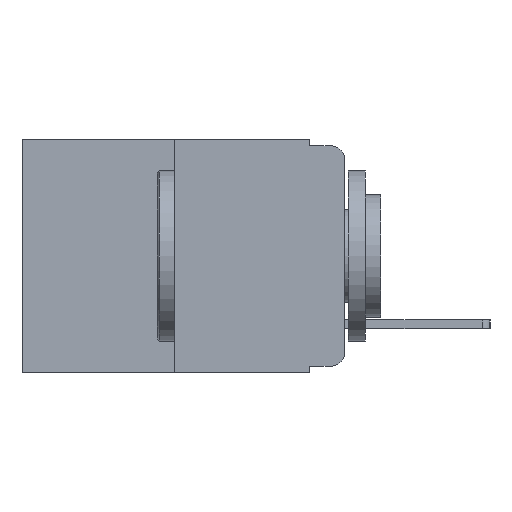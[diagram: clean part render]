
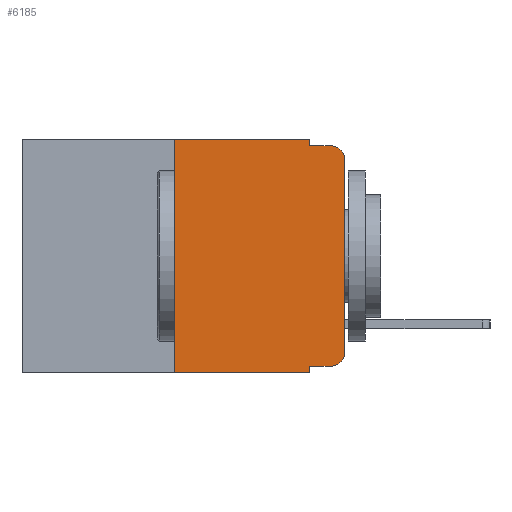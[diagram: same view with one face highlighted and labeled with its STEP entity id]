
A CAD part, left-side view. The second image highlights one B-rep face of the part: STEP entity #6185.
In plain terms, the highlighted planar face has unit normal (-1, 0, 0).
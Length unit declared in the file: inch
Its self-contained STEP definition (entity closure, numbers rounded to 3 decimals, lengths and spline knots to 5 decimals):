
#633 = CARTESIAN_POINT ( 'NONE',  ( 0., 0.02, -0.333 ) ) ;
#1030 = LINE ( 'NONE', #1947, #7232 ) ;
#1222 = CARTESIAN_POINT ( 'NONE',  ( 0., 0.02, -0.01 ) ) ;
#1385 = DIRECTION ( 'NONE',  ( 0., -1., 0. ) ) ;
#1588 = DIRECTION ( 'NONE',  ( 0., -1., 0. ) ) ;
#1858 = DIRECTION ( 'NONE',  ( 0., 0., -1. ) ) ;
#1947 = CARTESIAN_POINT ( 'NONE',  ( 0., 0.25, 0. ) ) ;
#2314 = CARTESIAN_POINT ( 'NONE',  ( 0., 0.051, 0. ) ) ;
#2353 = CARTESIAN_POINT ( 'NONE',  ( 0., 0.473, -0.343 ) ) ;
#2413 = CARTESIAN_POINT ( 'NONE',  ( 0., 0.051, -0.01 ) ) ;
#2487 = VERTEX_POINT ( 'NONE', #8614 ) ;
#2518 = CARTESIAN_POINT ( 'NONE',  ( 0., 0.02, -0.313 ) ) ;
#2602 = EDGE_CURVE ( 'NONE', #9831, #6729, #14370, .T. ) ;
#2634 = DIRECTION ( 'NONE',  ( -1., 0., 0. ) ) ;
#2783 = VECTOR ( 'NONE', #8376, 39.37008 ) ;
#2996 = LINE ( 'NONE', #5252, #14805 ) ;
#3298 = AXIS2_PLACEMENT_3D ( 'NONE', #2518, #2634, #12240 ) ;
#3332 = VERTEX_POINT ( 'NONE', #9084 ) ;
#3408 = EDGE_CURVE ( 'NONE', #10730, #9831, #14870, .T. ) ;
#3501 = ORIENTED_EDGE ( 'NONE', *, *, #6015, .F. ) ;
#4038 = FACE_OUTER_BOUND ( 'NONE', #9594, .T. ) ;
#4113 = CARTESIAN_POINT ( 'NONE',  ( 0., 0.051, -0.01 ) ) ;
#4253 = LINE ( 'NONE', #12933, #9910 ) ;
#4296 = EDGE_CURVE ( 'NONE', #10730, #9423, #14540, .T. ) ;
#5159 = EDGE_CURVE ( 'NONE', #3332, #11964, #1030, .T. ) ;
#5252 = CARTESIAN_POINT ( 'NONE',  ( 0., 0.473, 0. ) ) ;
#5679 = VERTEX_POINT ( 'NONE', #4113 ) ;
#5720 = ORIENTED_EDGE ( 'NONE', *, *, #6853, .F. ) ;
#6015 = EDGE_CURVE ( 'NONE', #11381, #5679, #4253, .T. ) ;
#6024 = DIRECTION ( 'NONE',  ( 0., 0., -1. ) ) ;
#6185 = ADVANCED_FACE ( 'NONE', ( #4038 ), #11193, .F. ) ;
#6373 = CARTESIAN_POINT ( 'NONE',  ( 0., 0.051, 0. ) ) ;
#6708 = DIRECTION ( 'NONE',  ( 0., 0., -1. ) ) ;
#6729 = VERTEX_POINT ( 'NONE', #9430 ) ;
#6853 = EDGE_CURVE ( 'NONE', #5679, #14169, #11876, .T. ) ;
#6919 = ORIENTED_EDGE ( 'NONE', *, *, #13422, .F. ) ;
#7162 = CARTESIAN_POINT ( 'NONE',  ( 0., 0.02, -0.03 ) ) ;
#7232 = VECTOR ( 'NONE', #11423, 39.37008 ) ;
#7352 = CARTESIAN_POINT ( 'NONE',  ( 0., 0.051, -0.343 ) ) ;
#7435 = DIRECTION ( 'NONE',  ( 0., -1., 0. ) ) ;
#7675 = EDGE_CURVE ( 'NONE', #2487, #14169, #11863, .T. ) ;
#8031 = ORIENTED_EDGE ( 'NONE', *, *, #3408, .T. ) ;
#8367 = LINE ( 'NONE', #2353, #10963 ) ;
#8376 = DIRECTION ( 'NONE',  ( 0., 0., 1. ) ) ;
#8444 = EDGE_CURVE ( 'NONE', #6729, #2487, #10025, .T. ) ;
#8569 = DIRECTION ( 'NONE',  ( 0., -1., 0. ) ) ;
#8614 = CARTESIAN_POINT ( 'NONE',  ( 0., 0., -0.03 ) ) ;
#8658 = VECTOR ( 'NONE', #7435, 39.37008 ) ;
#8742 = AXIS2_PLACEMENT_3D ( 'NONE', #7162, #9167, #1858 ) ;
#8881 = VECTOR ( 'NONE', #6024, 39.37008 ) ;
#9084 = CARTESIAN_POINT ( 'NONE',  ( 0., 0.25, -0.343 ) ) ;
#9167 = DIRECTION ( 'NONE',  ( -1., 0., 0. ) ) ;
#9423 = VERTEX_POINT ( 'NONE', #7352 ) ;
#9430 = CARTESIAN_POINT ( 'NONE',  ( 0., 0., -0.313 ) ) ;
#9463 = ORIENTED_EDGE ( 'NONE', *, *, #2602, .T. ) ;
#9594 = EDGE_LOOP ( 'NONE', ( #11141, #11462, #5720, #3501, #6919, #12809, #10321, #10660, #8031, #9463 ) ) ;
#9831 = VERTEX_POINT ( 'NONE', #633 ) ;
#9910 = VECTOR ( 'NONE', #13965, 39.37008 ) ;
#10025 = LINE ( 'NONE', #12695, #2783 ) ;
#10321 = ORIENTED_EDGE ( 'NONE', *, *, #11113, .T. ) ;
#10660 = ORIENTED_EDGE ( 'NONE', *, *, #4296, .F. ) ;
#10730 = VERTEX_POINT ( 'NONE', #12453 ) ;
#10963 = VECTOR ( 'NONE', #8569, 39.37008 ) ;
#11113 = EDGE_CURVE ( 'NONE', #3332, #9423, #8367, .T. ) ;
#11141 = ORIENTED_EDGE ( 'NONE', *, *, #8444, .T. ) ;
#11193 = PLANE ( 'NONE',  #14756 ) ;
#11381 = VERTEX_POINT ( 'NONE', #6373 ) ;
#11423 = DIRECTION ( 'NONE',  ( 0., 0., 1. ) ) ;
#11439 = VECTOR ( 'NONE', #1385, 39.37008 ) ;
#11462 = ORIENTED_EDGE ( 'NONE', *, *, #7675, .T. ) ;
#11863 = CIRCLE ( 'NONE', #8742, 0.02 ) ;
#11876 = LINE ( 'NONE', #2413, #8658 ) ;
#11964 = VERTEX_POINT ( 'NONE', #12277 ) ;
#12240 = DIRECTION ( 'NONE',  ( 0., 0., -1. ) ) ;
#12266 = CARTESIAN_POINT ( 'NONE',  ( 0., 0.473, 0. ) ) ;
#12277 = CARTESIAN_POINT ( 'NONE',  ( 0., 0.25, 0. ) ) ;
#12453 = CARTESIAN_POINT ( 'NONE',  ( 0., 0.051, -0.333 ) ) ;
#12695 = CARTESIAN_POINT ( 'NONE',  ( 0., 0., 0. ) ) ;
#12712 = CARTESIAN_POINT ( 'NONE',  ( 0., 0.051, -0.333 ) ) ;
#12809 = ORIENTED_EDGE ( 'NONE', *, *, #5159, .F. ) ;
#12933 = CARTESIAN_POINT ( 'NONE',  ( 0., 0.051, 0. ) ) ;
#13334 = DIRECTION ( 'NONE',  ( 1., 0., 0. ) ) ;
#13422 = EDGE_CURVE ( 'NONE', #11964, #11381, #2996, .T. ) ;
#13965 = DIRECTION ( 'NONE',  ( 0., 0., -1. ) ) ;
#14169 = VERTEX_POINT ( 'NONE', #1222 ) ;
#14370 = CIRCLE ( 'NONE', #3298, 0.02 ) ;
#14540 = LINE ( 'NONE', #2314, #8881 ) ;
#14756 = AXIS2_PLACEMENT_3D ( 'NONE', #12266, #13334, #6708 ) ;
#14805 = VECTOR ( 'NONE', #1588, 39.37008 ) ;
#14870 = LINE ( 'NONE', #12712, #11439 ) ;
